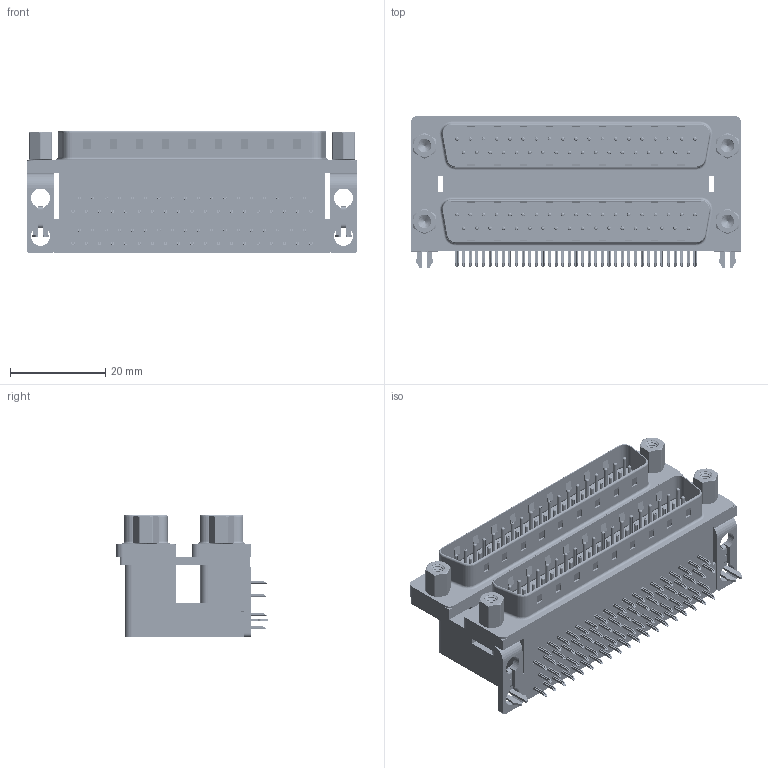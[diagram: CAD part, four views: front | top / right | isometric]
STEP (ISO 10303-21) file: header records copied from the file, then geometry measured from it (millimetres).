
FILE_DESCRIPTION (( 'STEP AP203' ), '1' );
FILE_NAME ('661-037-364-043.STEP', '2022-06-14T20:40:02', ( '' ), ( '' ), 'SwSTEP 2.0', 'SolidWorks 2020', '' );
FILE_SCHEMA (( 'CONFIG_CONTROL_DESIGN' ));
Length unit declared in the file: millimetre
Products named in the file (13): 661-037-364-043; 661 2 Prong Board Lock_4; 661 Threaded Rivet_4-40; 661 Contact Top Lower; 661 Contact Top Upper_L; 661 Shell_37 Contacts; 661 Housing Lower_37 Contacts; 661 4-40 Hex Standoff 5; 661 Mounting Bracket_2ProngL; 661 Contact Bottom Lower; 661 Contact Bottom Upper_L; 661 Housing Spacer_37 Contacts L; 661 Housing Upper_37 Contacts L
Assembly tree (91 placements, depth 2):
  661-037-364-043
    661 Housing Lower_37 Contacts
    661 Housing Spacer_37 Contacts L
    661 Housing Upper_37 Contacts L
    661 Shell_37 Contacts  x2
    661 Contact Bottom Lower  x18
    661 Contact Top Lower  x19
    661 Contact Bottom Upper_L  x18
    661 Contact Top Upper_L  x19
    661 Mounting Bracket_2ProngL  x2
    661 2 Prong Board Lock_4  x2
    661 Threaded Rivet_4-40  x4
    661 4-40 Hex Standoff 5  x4
Bounding box: 69.32 x 31.93 x 25.6 mm (x, y, z)
Volume: 28354.3 mm3; surface area: 29684.2 mm2
Topology: 91 solids, 91 shells, 6942 faces, 17338 edges, 10750 vertices
Faces by surface type: plane 4372, cylinder 1968, torus 506, cone 60, bspline 36
Entity records: 57410 total; most frequent: CARTESIAN_POINT 13323, ORIENTED_EDGE 8294, DIRECTION 8279, EDGE_CURVE 4147, LINE 3175, VECTOR 3175, VERTEX_POINT 2697, AXIS2_PLACEMENT_3D 2552
